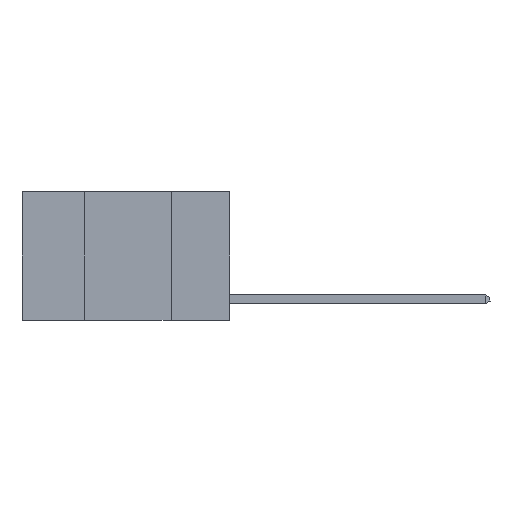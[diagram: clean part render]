
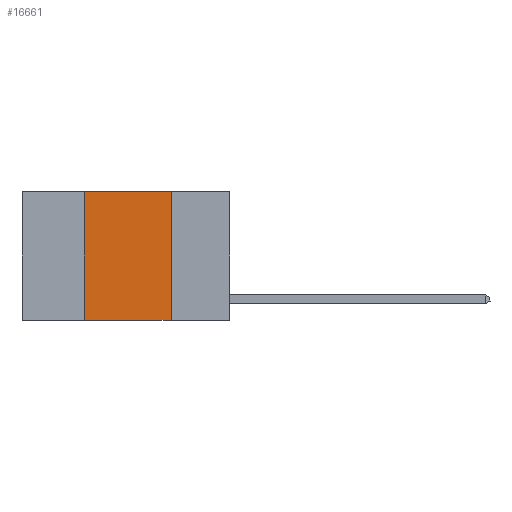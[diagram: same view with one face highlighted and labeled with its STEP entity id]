
A CAD part, left-side view. The second image highlights one B-rep face of the part: STEP entity #16661.
In plain terms, the highlighted planar face has unit normal (-1, 0, 0).
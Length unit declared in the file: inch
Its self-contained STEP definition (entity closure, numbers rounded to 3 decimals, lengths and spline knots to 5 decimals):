
#59 = VECTOR ( 'NONE', #23901, 39.37008 ) ;
#846 = DIRECTION ( 'NONE',  ( 1., 0., 0. ) ) ;
#2192 = VECTOR ( 'NONE', #11538, 39.37008 ) ;
#2598 = VERTEX_POINT ( 'NONE', #16818 ) ;
#2640 = CARTESIAN_POINT ( 'NONE',  ( 0., 0.42, 0. ) ) ;
#2906 = DIRECTION ( 'NONE',  ( 0., -1., 0. ) ) ;
#3146 = ORIENTED_EDGE ( 'NONE', *, *, #18781, .F. ) ;
#6557 = VERTEX_POINT ( 'NONE', #16042 ) ;
#7067 = VECTOR ( 'NONE', #16271, 39.37008 ) ;
#7237 = VERTEX_POINT ( 'NONE', #2640 ) ;
#7706 = LINE ( 'NONE', #21756, #7067 ) ;
#7765 = ORIENTED_EDGE ( 'NONE', *, *, #22269, .F. ) ;
#7840 = FACE_OUTER_BOUND ( 'NONE', #24648, .T. ) ;
#8972 = VECTOR ( 'NONE', #2906, 39.37008 ) ;
#9576 = CARTESIAN_POINT ( 'NONE',  ( 0., 0.6, -0.37 ) ) ;
#10699 = AXIS2_PLACEMENT_3D ( 'NONE', #12535, #846, #14435 ) ;
#11538 = DIRECTION ( 'NONE',  ( 0., -1., 0. ) ) ;
#12535 = CARTESIAN_POINT ( 'NONE',  ( 0., 0.6, 0. ) ) ;
#12549 = LINE ( 'NONE', #9576, #2192 ) ;
#14435 = DIRECTION ( 'NONE',  ( 0., 0., -1. ) ) ;
#15559 = LINE ( 'NONE', #21969, #59 ) ;
#16042 = CARTESIAN_POINT ( 'NONE',  ( 0., 0.17, -0.37 ) ) ;
#16271 = DIRECTION ( 'NONE',  ( 0., 0., -1. ) ) ;
#16661 = ADVANCED_FACE ( 'NONE', ( #7840 ), #23936, .F. ) ;
#16818 = CARTESIAN_POINT ( 'NONE',  ( 0., 0.17, 0. ) ) ;
#18541 = ORIENTED_EDGE ( 'NONE', *, *, #20990, .F. ) ;
#18781 = EDGE_CURVE ( 'NONE', #7237, #2598, #24172, .T. ) ;
#19136 = ORIENTED_EDGE ( 'NONE', *, *, #19713, .T. ) ;
#19713 = EDGE_CURVE ( 'NONE', #22557, #6557, #12549, .T. ) ;
#20176 = CARTESIAN_POINT ( 'NONE',  ( 0., 0.6, 0. ) ) ;
#20990 = EDGE_CURVE ( 'NONE', #22557, #7237, #15559, .T. ) ;
#21756 = CARTESIAN_POINT ( 'NONE',  ( 0., 0.17, 0. ) ) ;
#21969 = CARTESIAN_POINT ( 'NONE',  ( 0., 0.42, 0. ) ) ;
#22269 = EDGE_CURVE ( 'NONE', #2598, #6557, #7706, .T. ) ;
#22557 = VERTEX_POINT ( 'NONE', #24765 ) ;
#23901 = DIRECTION ( 'NONE',  ( 0., 0., 1. ) ) ;
#23936 = PLANE ( 'NONE',  #10699 ) ;
#24172 = LINE ( 'NONE', #20176, #8972 ) ;
#24648 = EDGE_LOOP ( 'NONE', ( #7765, #3146, #18541, #19136 ) ) ;
#24765 = CARTESIAN_POINT ( 'NONE',  ( 0., 0.42, -0.37 ) ) ;
